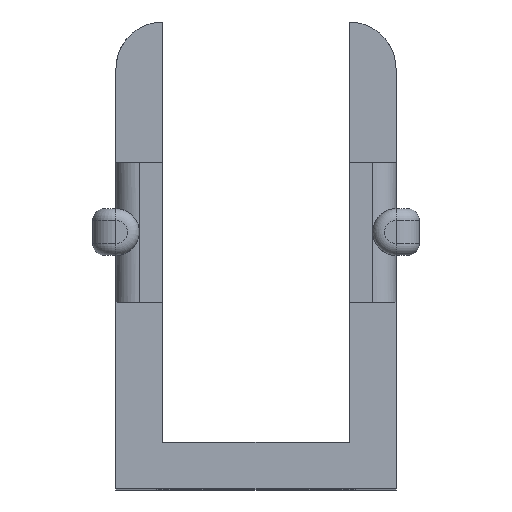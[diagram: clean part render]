
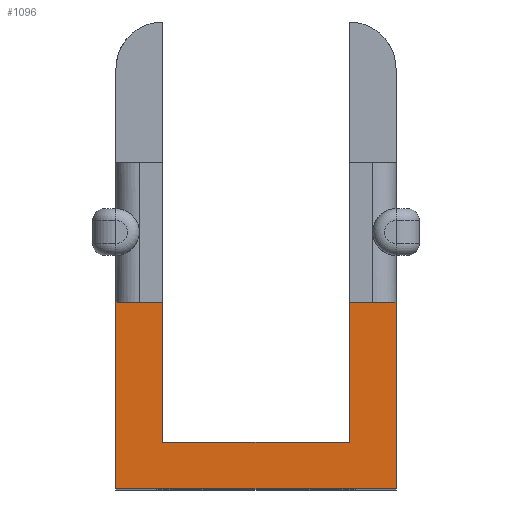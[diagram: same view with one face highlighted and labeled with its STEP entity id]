
A CAD part, top view. The second image highlights one B-rep face of the part: STEP entity #1096.
In plain terms, the highlighted planar face has unit normal (0, 0, 1).
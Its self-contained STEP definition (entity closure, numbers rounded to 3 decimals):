
#52 = DIRECTION ( 'NONE',  ( 1., 0., 0. ) ) ;
#80 = CARTESIAN_POINT ( 'NONE',  ( 0., -25., 80. ) ) ;
#93 = DIRECTION ( 'NONE',  ( 0., 1., 0. ) ) ;
#303 = DIRECTION ( 'NONE',  ( 0., -1., 0. ) ) ;
#450 = VECTOR ( 'NONE', #93, 1000. ) ;
#485 = EDGE_CURVE ( 'NONE', #3227, #1948, #2047, .T. ) ;
#555 = CARTESIAN_POINT ( 'NONE',  ( 25., -20., 80. ) ) ;
#615 = CARTESIAN_POINT ( 'NONE',  ( 5., -5., 80. ) ) ;
#646 = LINE ( 'NONE', #1634, #3306 ) ;
#851 = DIRECTION ( 'NONE',  ( 1., 0., 0. ) ) ;
#961 = EDGE_CURVE ( 'NONE', #1735, #3227, #2987, .T. ) ;
#1060 = CARTESIAN_POINT ( 'NONE',  ( 5., -20., 80. ) ) ;
#1096 = ADVANCED_FACE ( 'NONE', ( #2425 ), #3331, .F. ) ;
#1148 = VECTOR ( 'NONE', #52, 1000. ) ;
#1193 = VECTOR ( 'NONE', #851, 1000. ) ;
#1255 = ORIENTED_EDGE ( 'NONE', *, *, #961, .F. ) ;
#1292 = DIRECTION ( 'NONE',  ( 1., 0., 0. ) ) ;
#1296 = AXIS2_PLACEMENT_3D ( 'NONE', #3689, #1908, #3463 ) ;
#1329 = DIRECTION ( 'NONE',  ( 0., 1., 0. ) ) ;
#1330 = VECTOR ( 'NONE', #303, 1000. ) ;
#1334 = LINE ( 'NONE', #1438, #450 ) ;
#1435 = EDGE_CURVE ( 'NONE', #1735, #3329, #1334, .T. ) ;
#1438 = CARTESIAN_POINT ( 'NONE',  ( 5., -107.462, 80. ) ) ;
#1634 = CARTESIAN_POINT ( 'NONE',  ( 25., -5., 80. ) ) ;
#1644 = ORIENTED_EDGE ( 'NONE', *, *, #4379, .F. ) ;
#1648 = CARTESIAN_POINT ( 'NONE',  ( 25., -5., 80. ) ) ;
#1683 = VERTEX_POINT ( 'NONE', #2944 ) ;
#1735 = VERTEX_POINT ( 'NONE', #3220 ) ;
#1748 = VECTOR ( 'NONE', #2697, 1000. ) ;
#1768 = EDGE_CURVE ( 'NONE', #3172, #3329, #2091, .T. ) ;
#1797 = VERTEX_POINT ( 'NONE', #3640 ) ;
#1897 = EDGE_LOOP ( 'NONE', ( #1644, #2999, #2951, #1255, #2841, #4417, #2510, #3872 ) ) ;
#1908 = DIRECTION ( 'NONE',  ( 0., 0., -1. ) ) ;
#1921 = EDGE_CURVE ( 'NONE', #1948, #1683, #646, .T. ) ;
#1948 = VERTEX_POINT ( 'NONE', #1648 ) ;
#1975 = EDGE_CURVE ( 'NONE', #3172, #4357, #3199, .T. ) ;
#2010 = CARTESIAN_POINT ( 'NONE',  ( 30., -25., 80. ) ) ;
#2047 = LINE ( 'NONE', #3076, #2430 ) ;
#2091 = LINE ( 'NONE', #3264, #1193 ) ;
#2143 = DIRECTION ( 'NONE',  ( 0., -1., 0. ) ) ;
#2186 = CARTESIAN_POINT ( 'NONE',  ( 0., -5., 80. ) ) ;
#2425 = FACE_OUTER_BOUND ( 'NONE', #1897, .T. ) ;
#2430 = VECTOR ( 'NONE', #1329, 1000. ) ;
#2510 = ORIENTED_EDGE ( 'NONE', *, *, #1975, .T. ) ;
#2534 = LINE ( 'NONE', #3886, #3344 ) ;
#2697 = DIRECTION ( 'NONE',  ( -1., 0., 0. ) ) ;
#2740 = EDGE_CURVE ( 'NONE', #1797, #4357, #4390, .T. ) ;
#2841 = ORIENTED_EDGE ( 'NONE', *, *, #1435, .T. ) ;
#2944 = CARTESIAN_POINT ( 'NONE',  ( 30., -5., 80. ) ) ;
#2951 = ORIENTED_EDGE ( 'NONE', *, *, #485, .F. ) ;
#2987 = LINE ( 'NONE', #1060, #1148 ) ;
#2999 = ORIENTED_EDGE ( 'NONE', *, *, #1921, .F. ) ;
#3076 = CARTESIAN_POINT ( 'NONE',  ( 25., -107.462, 80. ) ) ;
#3172 = VERTEX_POINT ( 'NONE', #2186 ) ;
#3199 = LINE ( 'NONE', #4071, #1330 ) ;
#3220 = CARTESIAN_POINT ( 'NONE',  ( 5., -20., 80. ) ) ;
#3227 = VERTEX_POINT ( 'NONE', #555 ) ;
#3264 = CARTESIAN_POINT ( 'NONE',  ( 5., -5., 80. ) ) ;
#3306 = VECTOR ( 'NONE', #1292, 1000. ) ;
#3329 = VERTEX_POINT ( 'NONE', #615 ) ;
#3331 = PLANE ( 'NONE',  #1296 ) ;
#3344 = VECTOR ( 'NONE', #2143, 1000. ) ;
#3463 = DIRECTION ( 'NONE',  ( 0., 1., 0. ) ) ;
#3640 = CARTESIAN_POINT ( 'NONE',  ( 30., -25., 80. ) ) ;
#3689 = CARTESIAN_POINT ( 'NONE',  ( 30., 0., 80. ) ) ;
#3872 = ORIENTED_EDGE ( 'NONE', *, *, #2740, .F. ) ;
#3886 = CARTESIAN_POINT ( 'NONE',  ( 30., 0., 80. ) ) ;
#4071 = CARTESIAN_POINT ( 'NONE',  ( 0., 0., 80. ) ) ;
#4357 = VERTEX_POINT ( 'NONE', #80 ) ;
#4379 = EDGE_CURVE ( 'NONE', #1683, #1797, #2534, .T. ) ;
#4390 = LINE ( 'NONE', #2010, #1748 ) ;
#4417 = ORIENTED_EDGE ( 'NONE', *, *, #1768, .F. ) ;
